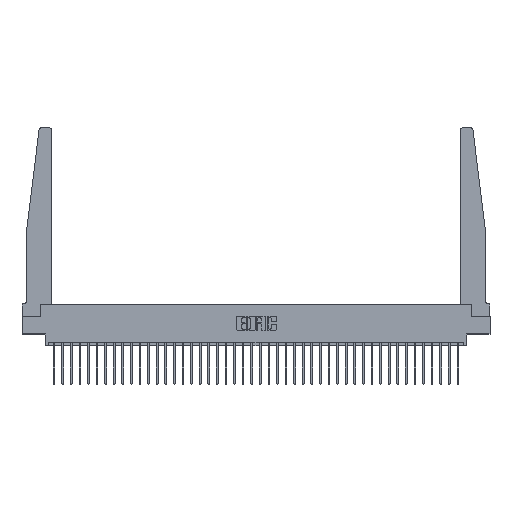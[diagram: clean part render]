
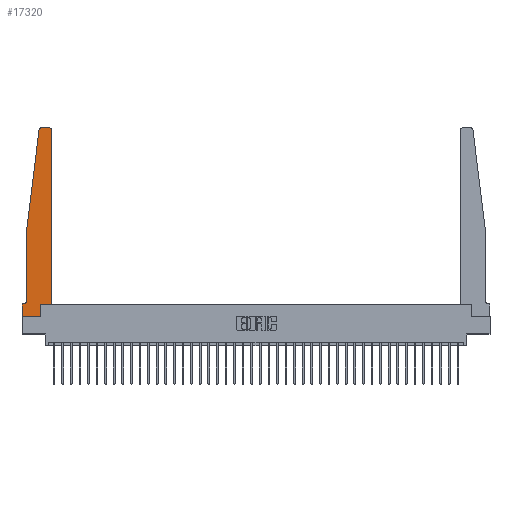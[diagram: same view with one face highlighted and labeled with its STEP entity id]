
A CAD part, top view. The second image highlights one B-rep face of the part: STEP entity #17320.
In plain terms, the highlighted planar face has unit normal (0, 0, 1).
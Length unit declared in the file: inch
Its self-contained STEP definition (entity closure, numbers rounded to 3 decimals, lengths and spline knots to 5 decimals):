
#120 = ORIENTED_EDGE ( 'NONE', *, *, #29679, .T. ) ;
#289 = ORIENTED_EDGE ( 'NONE', *, *, #28072, .T. ) ;
#970 = VECTOR ( 'NONE', #29309, 39.37008 ) ;
#1739 = EDGE_CURVE ( 'NONE', #13021, #17810, #28165, .T. ) ;
#2325 = CARTESIAN_POINT ( 'NONE',  ( 0.015, 0.1875, 0.37 ) ) ;
#2852 = CARTESIAN_POINT ( 'NONE',  ( 0.065, 0.2375, 0.37 ) ) ;
#3097 = LINE ( 'NONE', #10412, #16807 ) ;
#3488 = VERTEX_POINT ( 'NONE', #2852 ) ;
#3845 = EDGE_LOOP ( 'NONE', ( #25872, #32598, #120, #5741, #7194, #10517, #25626, #5912, #18430, #289, #33702, #9332 ) ) ;
#4016 = DIRECTION ( 'NONE',  ( 0., 0., 1. ) ) ;
#4194 = CARTESIAN_POINT ( 'NONE',  ( 0.065, 1.25, 0.37 ) ) ;
#4838 = DIRECTION ( 'NONE',  ( -1., 0., 0. ) ) ;
#5741 = ORIENTED_EDGE ( 'NONE', *, *, #31976, .T. ) ;
#5912 = ORIENTED_EDGE ( 'NONE', *, *, #1739, .T. ) ;
#6376 = VECTOR ( 'NONE', #21603, 39.37008 ) ;
#6803 = DIRECTION ( 'NONE',  ( 0., 0., 1. ) ) ;
#7111 = AXIS2_PLACEMENT_3D ( 'NONE', #24648, #8274, #27376 ) ;
#7194 = ORIENTED_EDGE ( 'NONE', *, *, #24847, .T. ) ;
#7324 = LINE ( 'NONE', #24338, #20977 ) ;
#7356 = VERTEX_POINT ( 'NONE', #21479 ) ;
#7388 = CARTESIAN_POINT ( 'NONE',  ( 0.065, 1.25, 0.37 ) ) ;
#8274 = DIRECTION ( 'NONE',  ( 0., 0., 1. ) ) ;
#8366 = AXIS2_PLACEMENT_3D ( 'NONE', #17671, #6803, #25921 ) ;
#8426 = EDGE_CURVE ( 'NONE', #15076, #13021, #22847, .T. ) ;
#9007 = DIRECTION ( 'NONE',  ( -0.122, -0.992, 0. ) ) ;
#9332 = ORIENTED_EDGE ( 'NONE', *, *, #23000, .T. ) ;
#9430 = PLANE ( 'NONE',  #8366 ) ;
#10326 = LINE ( 'NONE', #20159, #31230 ) ;
#10412 = CARTESIAN_POINT ( 'NONE',  ( 0.425, 0.18, 0.37 ) ) ;
#10472 = CARTESIAN_POINT ( 'NONE',  ( 0.395, 2.75, 0.37 ) ) ;
#10517 = ORIENTED_EDGE ( 'NONE', *, *, #14996, .T. ) ;
#10717 = LINE ( 'NONE', #25364, #26118 ) ;
#12267 = VECTOR ( 'NONE', #4838, 39.37008 ) ;
#13021 = VERTEX_POINT ( 'NONE', #15022 ) ;
#13145 = DIRECTION ( 'NONE',  ( 1., 0., 0. ) ) ;
#13193 = VERTEX_POINT ( 'NONE', #7388 ) ;
#13362 = CARTESIAN_POINT ( 'NONE',  ( 0., 0., 0.37 ) ) ;
#13407 = EDGE_CURVE ( 'NONE', #15092, #27307, #20669, .T. ) ;
#13451 = DIRECTION ( 'NONE',  ( 0., 0., -1. ) ) ;
#14527 = CARTESIAN_POINT ( 'NONE',  ( 0.2605, 0.18, 0.37 ) ) ;
#14686 = AXIS2_PLACEMENT_3D ( 'NONE', #29805, #13451, #32546 ) ;
#14996 = EDGE_CURVE ( 'NONE', #19279, #15076, #7324, .T. ) ;
#15022 = CARTESIAN_POINT ( 'NONE',  ( 0., 0., 0.37 ) ) ;
#15076 = VERTEX_POINT ( 'NONE', #22216 ) ;
#15092 = VERTEX_POINT ( 'NONE', #24978 ) ;
#15725 = CARTESIAN_POINT ( 'NONE',  ( 0.25, 2.75, 0.37 ) ) ;
#16043 = LINE ( 'NONE', #4194, #21562 ) ;
#16807 = VECTOR ( 'NONE', #13145, 39.37008 ) ;
#17320 = ADVANCED_FACE ( 'NONE', ( #28126 ), #9430, .T. ) ;
#17647 = CARTESIAN_POINT ( 'NONE',  ( 0.2605, 0., 0.37 ) ) ;
#17671 = CARTESIAN_POINT ( 'NONE',  ( 0., 0.1875, 0.37 ) ) ;
#17810 = VERTEX_POINT ( 'NONE', #17647 ) ;
#18044 = EDGE_CURVE ( 'NONE', #19932, #7356, #26808, .T. ) ;
#18245 = CARTESIAN_POINT ( 'NONE',  ( 0.425, 2.72, 0.37 ) ) ;
#18430 = ORIENTED_EDGE ( 'NONE', *, *, #21894, .T. ) ;
#19279 = VERTEX_POINT ( 'NONE', #2325 ) ;
#19932 = VERTEX_POINT ( 'NONE', #10472 ) ;
#20159 = CARTESIAN_POINT ( 'NONE',  ( 0.2605, 0.18, 0.37 ) ) ;
#20387 = VERTEX_POINT ( 'NONE', #20702 ) ;
#20417 = CARTESIAN_POINT ( 'NONE',  ( 0.27653, 2.72, 0.37 ) ) ;
#20669 = LINE ( 'NONE', #30268, #27085 ) ;
#20702 = CARTESIAN_POINT ( 'NONE',  ( 0.24675, 2.72367, 0.37 ) ) ;
#20977 = VECTOR ( 'NONE', #21564, 39.37008 ) ;
#21479 = CARTESIAN_POINT ( 'NONE',  ( 0.27653, 2.75, 0.37 ) ) ;
#21562 = VECTOR ( 'NONE', #28814, 39.37008 ) ;
#21564 = DIRECTION ( 'NONE',  ( -1., 0., 0. ) ) ;
#21603 = DIRECTION ( 'NONE',  ( 1., 0., 0. ) ) ;
#21894 = EDGE_CURVE ( 'NONE', #17810, #27050, #10326, .T. ) ;
#22042 = DIRECTION ( 'NONE',  ( 0., 1., 0. ) ) ;
#22216 = CARTESIAN_POINT ( 'NONE',  ( 0., 0.1875, 0.37 ) ) ;
#22847 = LINE ( 'NONE', #26588, #970 ) ;
#22902 = DIRECTION ( 'NONE',  ( 0., 1., 0. ) ) ;
#23000 = EDGE_CURVE ( 'NONE', #27307, #19932, #33297, .T. ) ;
#23153 = DIRECTION ( 'NONE',  ( 1., 0., 0. ) ) ;
#24338 = CARTESIAN_POINT ( 'NONE',  ( 0.065, 0.1875, 0.37 ) ) ;
#24648 = CARTESIAN_POINT ( 'NONE',  ( 0.395, 2.72, 0.37 ) ) ;
#24847 = EDGE_CURVE ( 'NONE', #3488, #19279, #28516, .T. ) ;
#24978 = CARTESIAN_POINT ( 'NONE',  ( 0.425, 0.18, 0.37 ) ) ;
#25364 = CARTESIAN_POINT ( 'NONE',  ( 0.065, 1.25, 0.37 ) ) ;
#25626 = ORIENTED_EDGE ( 'NONE', *, *, #8426, .T. ) ;
#25771 = CIRCLE ( 'NONE', #29828, 0.03 ) ;
#25872 = ORIENTED_EDGE ( 'NONE', *, *, #18044, .T. ) ;
#25921 = DIRECTION ( 'NONE',  ( 1., 0., 0. ) ) ;
#26118 = VECTOR ( 'NONE', #9007, 39.37008 ) ;
#26588 = CARTESIAN_POINT ( 'NONE',  ( 0., 0., 0.37 ) ) ;
#26808 = LINE ( 'NONE', #15725, #12267 ) ;
#27050 = VERTEX_POINT ( 'NONE', #14527 ) ;
#27085 = VECTOR ( 'NONE', #22042, 39.37008 ) ;
#27307 = VERTEX_POINT ( 'NONE', #18245 ) ;
#27376 = DIRECTION ( 'NONE',  ( 1., 0., 0. ) ) ;
#28072 = EDGE_CURVE ( 'NONE', #27050, #15092, #3097, .T. ) ;
#28126 = FACE_OUTER_BOUND ( 'NONE', #3845, .T. ) ;
#28165 = LINE ( 'NONE', #13362, #6376 ) ;
#28498 = EDGE_CURVE ( 'NONE', #7356, #20387, #25771, .T. ) ;
#28516 = CIRCLE ( 'NONE', #14686, 0.05 ) ;
#28814 = DIRECTION ( 'NONE',  ( 0., -1., 0. ) ) ;
#29309 = DIRECTION ( 'NONE',  ( 0., -1., 0. ) ) ;
#29679 = EDGE_CURVE ( 'NONE', #20387, #13193, #10717, .T. ) ;
#29805 = CARTESIAN_POINT ( 'NONE',  ( 0.015, 0.2375, 0.37 ) ) ;
#29828 = AXIS2_PLACEMENT_3D ( 'NONE', #20417, #4016, #23153 ) ;
#30268 = CARTESIAN_POINT ( 'NONE',  ( 0.425, 0.18, 0.37 ) ) ;
#31230 = VECTOR ( 'NONE', #22902, 39.37008 ) ;
#31976 = EDGE_CURVE ( 'NONE', #13193, #3488, #16043, .T. ) ;
#32546 = DIRECTION ( 'NONE',  ( -1., 0., 0. ) ) ;
#32598 = ORIENTED_EDGE ( 'NONE', *, *, #28498, .T. ) ;
#33297 = CIRCLE ( 'NONE', #7111, 0.03 ) ;
#33702 = ORIENTED_EDGE ( 'NONE', *, *, #13407, .T. ) ;
